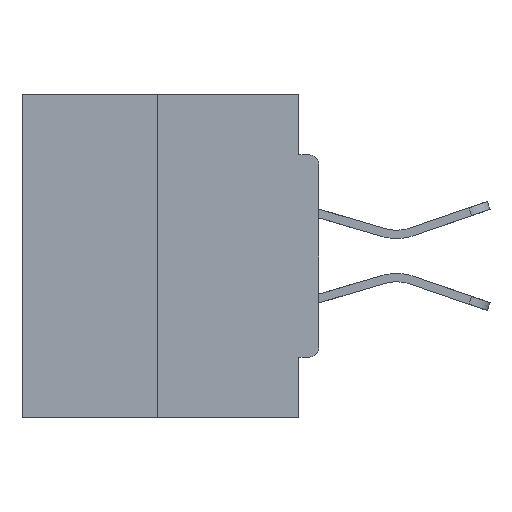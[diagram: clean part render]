
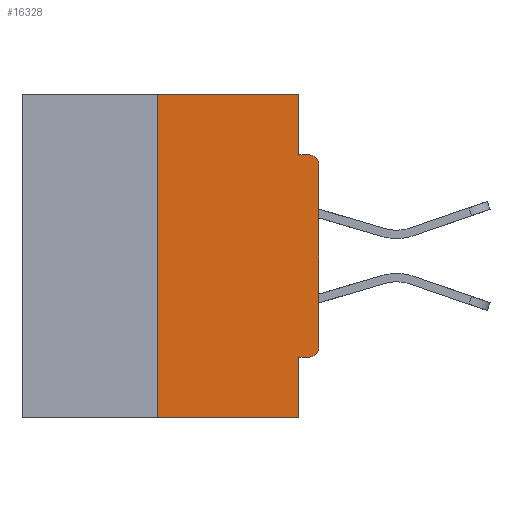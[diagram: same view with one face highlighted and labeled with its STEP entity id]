
A CAD part, left-side view. The second image highlights one B-rep face of the part: STEP entity #16328.
In plain terms, the highlighted planar face has unit normal (-1, 0, 0).
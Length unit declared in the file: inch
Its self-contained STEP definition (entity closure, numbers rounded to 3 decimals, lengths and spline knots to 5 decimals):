
#89 = CARTESIAN_POINT ( 'NONE',  ( 0., 0., 0. ) ) ;
#221 = ORIENTED_EDGE ( 'NONE', *, *, #21178, .F. ) ;
#619 = DIRECTION ( 'NONE',  ( 0., 0., -1. ) ) ;
#634 = ORIENTED_EDGE ( 'NONE', *, *, #18598, .F. ) ;
#690 = VERTEX_POINT ( 'NONE', #20994 ) ;
#750 = VECTOR ( 'NONE', #4080, 39.37008 ) ;
#1072 = DIRECTION ( 'NONE',  ( 1., 0., 0. ) ) ;
#1819 = VECTOR ( 'NONE', #15894, 39.37008 ) ;
#2001 = CARTESIAN_POINT ( 'NONE',  ( 0., 0.25, 0. ) ) ;
#3054 = FACE_OUTER_BOUND ( 'NONE', #23461, .T. ) ;
#4054 = ORIENTED_EDGE ( 'NONE', *, *, #5680, .F. ) ;
#4080 = DIRECTION ( 'NONE',  ( 0., 0., 1. ) ) ;
#4083 = CIRCLE ( 'NONE', #21439, 0.015 ) ;
#4125 = VERTEX_POINT ( 'NONE', #20318 ) ;
#5107 = VECTOR ( 'NONE', #619, 39.37008 ) ;
#5241 = VECTOR ( 'NONE', #27249, 39.37008 ) ;
#5653 = CARTESIAN_POINT ( 'NONE',  ( 0., 0.031, 0. ) ) ;
#5680 = EDGE_CURVE ( 'NONE', #23181, #12037, #18024, .T. ) ;
#5693 = ORIENTED_EDGE ( 'NONE', *, *, #26997, .F. ) ;
#5762 = VERTEX_POINT ( 'NONE', #26339 ) ;
#6793 = LINE ( 'NONE', #24946, #5241 ) ;
#7171 = CARTESIAN_POINT ( 'NONE',  ( 0., 0.25, -0.5 ) ) ;
#8181 = VERTEX_POINT ( 'NONE', #9439 ) ;
#9439 = CARTESIAN_POINT ( 'NONE',  ( 0., 0., -0.1085 ) ) ;
#9457 = EDGE_CURVE ( 'NONE', #24678, #22126, #4083, .T. ) ;
#9738 = DIRECTION ( 'NONE',  ( 0., -1., 0. ) ) ;
#10370 = LINE ( 'NONE', #17728, #20271 ) ;
#10889 = EDGE_CURVE ( 'NONE', #22126, #8181, #28558, .T. ) ;
#11112 = ORIENTED_EDGE ( 'NONE', *, *, #25103, .F. ) ;
#11203 = PLANE ( 'NONE',  #18152 ) ;
#12037 = VERTEX_POINT ( 'NONE', #23127 ) ;
#12755 = DIRECTION ( 'NONE',  ( 0., 1., 0. ) ) ;
#13416 = DIRECTION ( 'NONE',  ( 0., 0., -1. ) ) ;
#14410 = LINE ( 'NONE', #17713, #15582 ) ;
#14538 = CARTESIAN_POINT ( 'NONE',  ( 0., 0.031, -0.5 ) ) ;
#14618 = LINE ( 'NONE', #27474, #28445 ) ;
#15015 = CARTESIAN_POINT ( 'NONE',  ( 0., 0.015, -0.3915 ) ) ;
#15582 = VECTOR ( 'NONE', #27854, 39.37008 ) ;
#15709 = LINE ( 'NONE', #14538, #28340 ) ;
#15894 = DIRECTION ( 'NONE',  ( 0., 0., 1. ) ) ;
#16205 = CARTESIAN_POINT ( 'NONE',  ( 0., 0., -0.3915 ) ) ;
#16264 = AXIS2_PLACEMENT_3D ( 'NONE', #27072, #16628, #29630 ) ;
#16328 = ADVANCED_FACE ( 'NONE', ( #3054 ), #11203, .F. ) ;
#16485 = VERTEX_POINT ( 'NONE', #24128 ) ;
#16565 = ORIENTED_EDGE ( 'NONE', *, *, #19735, .T. ) ;
#16628 = DIRECTION ( 'NONE',  ( -1., 0., 0. ) ) ;
#17713 = CARTESIAN_POINT ( 'NONE',  ( 0., 0., -0.0935 ) ) ;
#17728 = CARTESIAN_POINT ( 'NONE',  ( 0., 0., -0.4065 ) ) ;
#18024 = LINE ( 'NONE', #5653, #5107 ) ;
#18073 = DIRECTION ( 'NONE',  ( -1., 0., 0. ) ) ;
#18152 = AXIS2_PLACEMENT_3D ( 'NONE', #23915, #1072, #13416 ) ;
#18598 = EDGE_CURVE ( 'NONE', #690, #23181, #6793, .T. ) ;
#19205 = VERTEX_POINT ( 'NONE', #7171 ) ;
#19222 = LINE ( 'NONE', #2001, #750 ) ;
#19735 = EDGE_CURVE ( 'NONE', #19205, #16485, #14618, .T. ) ;
#20271 = VECTOR ( 'NONE', #12755, 39.37008 ) ;
#20318 = CARTESIAN_POINT ( 'NONE',  ( 0., 0.015, -0.0935 ) ) ;
#20994 = CARTESIAN_POINT ( 'NONE',  ( 0., 0.25, 0. ) ) ;
#21178 = EDGE_CURVE ( 'NONE', #5762, #16485, #15709, .T. ) ;
#21439 = AXIS2_PLACEMENT_3D ( 'NONE', #15015, #18073, #27454 ) ;
#21590 = CARTESIAN_POINT ( 'NONE',  ( 0., 0.015, -0.4065 ) ) ;
#21820 = ORIENTED_EDGE ( 'NONE', *, *, #32356, .F. ) ;
#22126 = VERTEX_POINT ( 'NONE', #16205 ) ;
#22493 = ORIENTED_EDGE ( 'NONE', *, *, #10889, .T. ) ;
#23127 = CARTESIAN_POINT ( 'NONE',  ( 0., 0.031, -0.0935 ) ) ;
#23181 = VERTEX_POINT ( 'NONE', #30410 ) ;
#23461 = EDGE_LOOP ( 'NONE', ( #634, #11112, #16565, #221, #5693, #26534, #22493, #28304, #21820, #4054 ) ) ;
#23915 = CARTESIAN_POINT ( 'NONE',  ( 0., 0.46, 0. ) ) ;
#24128 = CARTESIAN_POINT ( 'NONE',  ( 0., 0.031, -0.5 ) ) ;
#24678 = VERTEX_POINT ( 'NONE', #21590 ) ;
#24946 = CARTESIAN_POINT ( 'NONE',  ( 0., 0.46, 0. ) ) ;
#25103 = EDGE_CURVE ( 'NONE', #19205, #690, #19222, .T. ) ;
#25487 = CIRCLE ( 'NONE', #16264, 0.015 ) ;
#25570 = EDGE_CURVE ( 'NONE', #8181, #4125, #25487, .T. ) ;
#26339 = CARTESIAN_POINT ( 'NONE',  ( 0., 0.031, -0.4065 ) ) ;
#26534 = ORIENTED_EDGE ( 'NONE', *, *, #9457, .T. ) ;
#26997 = EDGE_CURVE ( 'NONE', #24678, #5762, #10370, .T. ) ;
#27072 = CARTESIAN_POINT ( 'NONE',  ( 0., 0.015, -0.1085 ) ) ;
#27249 = DIRECTION ( 'NONE',  ( 0., -1., 0. ) ) ;
#27454 = DIRECTION ( 'NONE',  ( 0., 0., -1. ) ) ;
#27474 = CARTESIAN_POINT ( 'NONE',  ( 0., 0.46, -0.5 ) ) ;
#27854 = DIRECTION ( 'NONE',  ( 0., -1., 0. ) ) ;
#28304 = ORIENTED_EDGE ( 'NONE', *, *, #25570, .T. ) ;
#28340 = VECTOR ( 'NONE', #29232, 39.37008 ) ;
#28445 = VECTOR ( 'NONE', #9738, 39.37008 ) ;
#28558 = LINE ( 'NONE', #89, #1819 ) ;
#29232 = DIRECTION ( 'NONE',  ( 0., 0., -1. ) ) ;
#29630 = DIRECTION ( 'NONE',  ( 0., 0., -1. ) ) ;
#30410 = CARTESIAN_POINT ( 'NONE',  ( 0., 0.031, 0. ) ) ;
#32356 = EDGE_CURVE ( 'NONE', #12037, #4125, #14410, .T. ) ;
